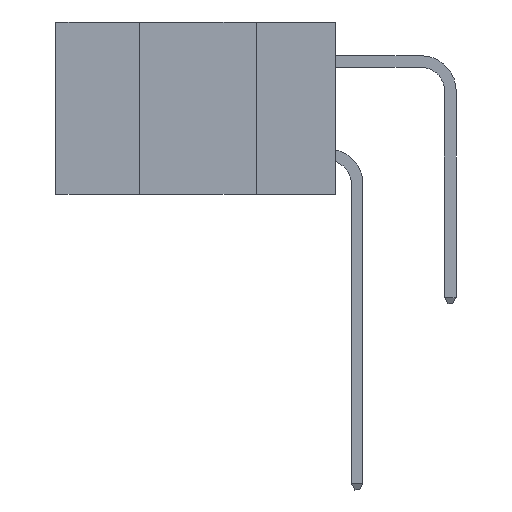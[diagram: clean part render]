
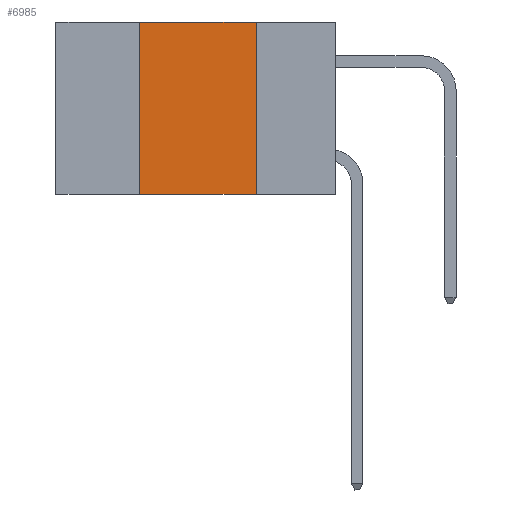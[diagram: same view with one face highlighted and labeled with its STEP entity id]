
A CAD part, left-side view. The second image highlights one B-rep face of the part: STEP entity #6985.
In plain terms, the highlighted planar face has unit normal (-1, 0, 0).
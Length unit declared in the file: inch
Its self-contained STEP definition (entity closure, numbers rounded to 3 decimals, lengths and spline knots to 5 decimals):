
#233 = EDGE_CURVE ( 'NONE', #7957, #12258, #8387, .T. ) ;
#1583 = CARTESIAN_POINT ( 'NONE',  ( 0., 0.17, -0.37 ) ) ;
#1738 = ORIENTED_EDGE ( 'NONE', *, *, #233, .F. ) ;
#2696 = EDGE_CURVE ( 'NONE', #12258, #5864, #12621, .T. ) ;
#3139 = CARTESIAN_POINT ( 'NONE',  ( 0., 0.42, -0.37 ) ) ;
#3235 = DIRECTION ( 'NONE',  ( 0., -1., 0. ) ) ;
#3267 = AXIS2_PLACEMENT_3D ( 'NONE', #11033, #5219, #11920 ) ;
#3460 = CARTESIAN_POINT ( 'NONE',  ( 0., 0.42, 0. ) ) ;
#3876 = VECTOR ( 'NONE', #3235, 39.37008 ) ;
#4048 = DIRECTION ( 'NONE',  ( 0., -1., 0. ) ) ;
#4984 = LINE ( 'NONE', #3460, #12333 ) ;
#5174 = PLANE ( 'NONE',  #3267 ) ;
#5219 = DIRECTION ( 'NONE',  ( 1., 0., 0. ) ) ;
#5419 = ORIENTED_EDGE ( 'NONE', *, *, #10560, .F. ) ;
#5671 = VECTOR ( 'NONE', #4048, 39.37008 ) ;
#5864 = VERTEX_POINT ( 'NONE', #1583 ) ;
#6268 = CARTESIAN_POINT ( 'NONE',  ( 0., 0.6, -0.37 ) ) ;
#6502 = DIRECTION ( 'NONE',  ( 0., 0., -1. ) ) ;
#6985 = ADVANCED_FACE ( 'NONE', ( #11305 ), #5174, .F. ) ;
#6988 = EDGE_CURVE ( 'NONE', #7475, #5864, #8899, .T. ) ;
#7122 = EDGE_LOOP ( 'NONE', ( #7678, #1738, #5419, #8895 ) ) ;
#7212 = CARTESIAN_POINT ( 'NONE',  ( 0., 0.17, 0. ) ) ;
#7475 = VERTEX_POINT ( 'NONE', #3139 ) ;
#7678 = ORIENTED_EDGE ( 'NONE', *, *, #2696, .F. ) ;
#7957 = VERTEX_POINT ( 'NONE', #10664 ) ;
#8387 = LINE ( 'NONE', #10611, #5671 ) ;
#8895 = ORIENTED_EDGE ( 'NONE', *, *, #6988, .T. ) ;
#8899 = LINE ( 'NONE', #6268, #3876 ) ;
#9320 = CARTESIAN_POINT ( 'NONE',  ( 0., 0.17, 0. ) ) ;
#10204 = VECTOR ( 'NONE', #6502, 39.37008 ) ;
#10320 = DIRECTION ( 'NONE',  ( 0., 0., 1. ) ) ;
#10560 = EDGE_CURVE ( 'NONE', #7475, #7957, #4984, .T. ) ;
#10611 = CARTESIAN_POINT ( 'NONE',  ( 0., 0.6, 0. ) ) ;
#10664 = CARTESIAN_POINT ( 'NONE',  ( 0., 0.42, 0. ) ) ;
#11033 = CARTESIAN_POINT ( 'NONE',  ( 0., 0.6, 0. ) ) ;
#11305 = FACE_OUTER_BOUND ( 'NONE', #7122, .T. ) ;
#11920 = DIRECTION ( 'NONE',  ( 0., 0., -1. ) ) ;
#12258 = VERTEX_POINT ( 'NONE', #9320 ) ;
#12333 = VECTOR ( 'NONE', #10320, 39.37008 ) ;
#12621 = LINE ( 'NONE', #7212, #10204 ) ;
